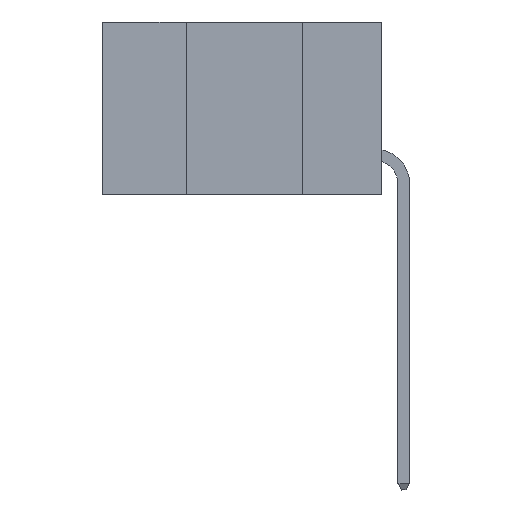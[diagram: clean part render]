
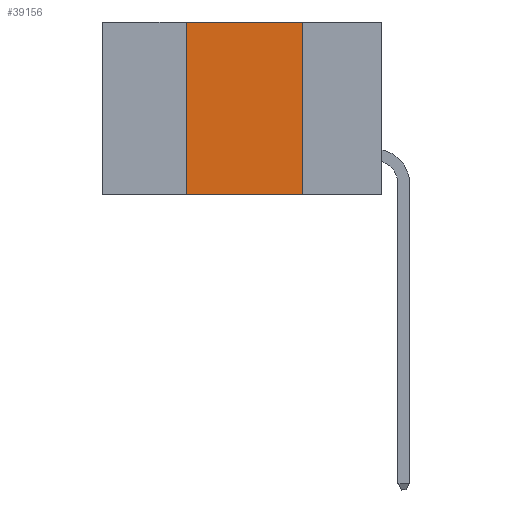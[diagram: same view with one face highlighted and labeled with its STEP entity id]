
A CAD part, left-side view. The second image highlights one B-rep face of the part: STEP entity #39156.
In plain terms, the highlighted planar face has unit normal (-1, 0, 0).
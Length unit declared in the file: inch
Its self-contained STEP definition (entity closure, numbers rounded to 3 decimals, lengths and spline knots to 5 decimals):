
#182 = ORIENTED_EDGE ( 'NONE', *, *, #12311, .F. ) ;
#639 = ORIENTED_EDGE ( 'NONE', *, *, #841, .T. ) ;
#841 = EDGE_CURVE ( 'NONE', #7984, #9941, #34141, .T. ) ;
#5235 = LINE ( 'NONE', #5765, #31796 ) ;
#5765 = CARTESIAN_POINT ( 'NONE',  ( 0., 0.17, 0. ) ) ;
#5766 = VECTOR ( 'NONE', #35947, 39.37008 ) ;
#7376 = VERTEX_POINT ( 'NONE', #18084 ) ;
#7984 = VERTEX_POINT ( 'NONE', #26622 ) ;
#9941 = VERTEX_POINT ( 'NONE', #39583 ) ;
#10547 = CARTESIAN_POINT ( 'NONE',  ( 0., 0.6, -0.37 ) ) ;
#11982 = EDGE_CURVE ( 'NONE', #13952, #9941, #5235, .T. ) ;
#12311 = EDGE_CURVE ( 'NONE', #7984, #7376, #43113, .T. ) ;
#13952 = VERTEX_POINT ( 'NONE', #17751 ) ;
#16921 = DIRECTION ( 'NONE',  ( 1., 0., 0. ) ) ;
#17751 = CARTESIAN_POINT ( 'NONE',  ( 0., 0.17, 0. ) ) ;
#18084 = CARTESIAN_POINT ( 'NONE',  ( 0., 0.42, 0. ) ) ;
#19891 = LINE ( 'NONE', #36274, #5766 ) ;
#23613 = FACE_OUTER_BOUND ( 'NONE', #43957, .T. ) ;
#26622 = CARTESIAN_POINT ( 'NONE',  ( 0., 0.42, -0.37 ) ) ;
#29225 = VECTOR ( 'NONE', #33930, 39.37008 ) ;
#30558 = EDGE_CURVE ( 'NONE', #7376, #13952, #19891, .T. ) ;
#31026 = PLANE ( 'NONE',  #43859 ) ;
#31756 = VECTOR ( 'NONE', #44705, 39.37008 ) ;
#31796 = VECTOR ( 'NONE', #36551, 39.37008 ) ;
#33930 = DIRECTION ( 'NONE',  ( 0., -1., 0. ) ) ;
#34141 = LINE ( 'NONE', #10547, #29225 ) ;
#34617 = CARTESIAN_POINT ( 'NONE',  ( 0., 0.6, 0. ) ) ;
#35947 = DIRECTION ( 'NONE',  ( 0., -1., 0. ) ) ;
#36274 = CARTESIAN_POINT ( 'NONE',  ( 0., 0.6, 0. ) ) ;
#36551 = DIRECTION ( 'NONE',  ( 0., 0., -1. ) ) ;
#38847 = ORIENTED_EDGE ( 'NONE', *, *, #30558, .F. ) ;
#39156 = ADVANCED_FACE ( 'NONE', ( #23613 ), #31026, .F. ) ;
#39583 = CARTESIAN_POINT ( 'NONE',  ( 0., 0.17, -0.37 ) ) ;
#40986 = CARTESIAN_POINT ( 'NONE',  ( 0., 0.42, 0. ) ) ;
#41143 = DIRECTION ( 'NONE',  ( 0., 0., -1. ) ) ;
#43113 = LINE ( 'NONE', #40986, #31756 ) ;
#43859 = AXIS2_PLACEMENT_3D ( 'NONE', #34617, #16921, #41143 ) ;
#43957 = EDGE_LOOP ( 'NONE', ( #44744, #38847, #182, #639 ) ) ;
#44705 = DIRECTION ( 'NONE',  ( 0., 0., 1. ) ) ;
#44744 = ORIENTED_EDGE ( 'NONE', *, *, #11982, .F. ) ;
